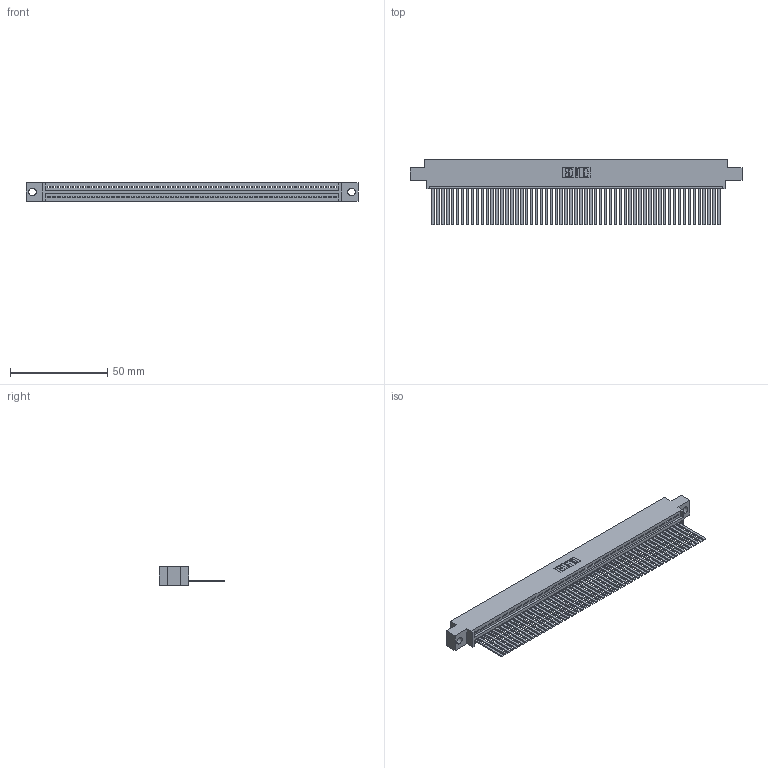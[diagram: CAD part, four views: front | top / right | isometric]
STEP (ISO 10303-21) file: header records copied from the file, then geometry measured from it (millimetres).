
FILE_DESCRIPTION (( 'STEP AP203' ), '1' );
FILE_NAME ('395-059-544-604.STEP', '2021-05-31T21:46:51', ( '' ), ( '' ), 'SwSTEP 2.0', 'SolidWorks 2020', '' );
FILE_SCHEMA (( 'CONFIG_CONTROL_DESIGN' ));
Length unit declared in the file: inch
Products named in the file (3): 345-292-001_345-293-144; 395-059-544-604; 345 Part_0.170 Offset - 0.156 Dia-TI
Assembly tree (60 placements, depth 2):
  395-059-544-604
    345 Part_0.170 Offset - 0.156 Dia-TI
    345-292-001_345-293-144  x59
Bounding box: 171.07 x 33.96 x 9.4 mm (x, y, z)
Volume: 16851.5 mm3; surface area: 24645.6 mm2
Topology: 60 solids, 60 shells, 3212 faces, 9711 edges, 6394 vertices
Faces by surface type: plane 2222, cylinder 990
Entity records: 42483 total; most frequent: CARTESIAN_POINT 7367, ORIENTED_EDGE 7358, DIRECTION 6405, EDGE_CURVE 3679, LINE 3315, VECTOR 3315, VERTEX_POINT 2450, AXIS2_PLACEMENT_3D 1545
